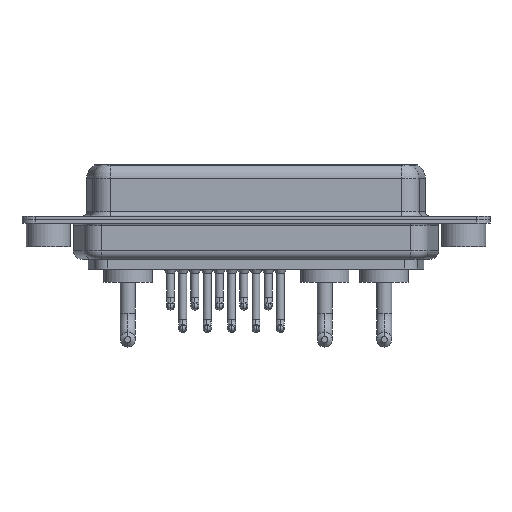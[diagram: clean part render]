
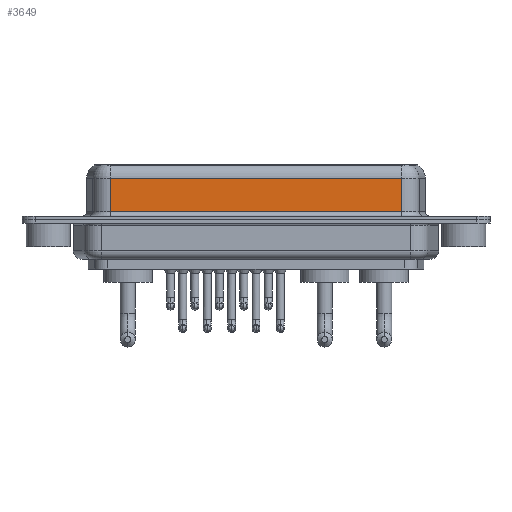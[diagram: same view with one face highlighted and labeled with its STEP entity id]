
A CAD part, front view. The second image highlights one B-rep face of the part: STEP entity #3649.
In plain terms, the highlighted planar face has unit normal (0, -1, 0).
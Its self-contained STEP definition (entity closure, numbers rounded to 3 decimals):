
#179 = LINE ( 'NONE', #17613, #16798 ) ;
#196 = VERTEX_POINT ( 'NONE', #9562 ) ;
#978 = CARTESIAN_POINT ( 'NONE',  ( 40.037, -3.95, 6.4 ) ) ;
#1635 = CARTESIAN_POINT ( 'NONE',  ( 40.037, -3.95, 4.65 ) ) ;
#2036 = ORIENTED_EDGE ( 'NONE', *, *, #8078, .T. ) ;
#2065 = ORIENTED_EDGE ( 'NONE', *, *, #15577, .F. ) ;
#2569 = CARTESIAN_POINT ( 'NONE',  ( 40.037, -3.95, 0.9 ) ) ;
#3183 = VECTOR ( 'NONE', #7528, 1000. ) ;
#3245 = EDGE_CURVE ( 'NONE', #16945, #6229, #15937, .T. ) ;
#3649 = ADVANCED_FACE ( 'NONE', ( #14176 ), #4058, .F. ) ;
#3755 = EDGE_CURVE ( 'NONE', #196, #16945, #179, .T. ) ;
#4058 = PLANE ( 'NONE',  #8174 ) ;
#5156 = ORIENTED_EDGE ( 'NONE', *, *, #3245, .T. ) ;
#5702 = VECTOR ( 'NONE', #10229, 1000. ) ;
#6049 = CARTESIAN_POINT ( 'NONE',  ( 7.013, -3.95, 0.9 ) ) ;
#6229 = VERTEX_POINT ( 'NONE', #11661 ) ;
#7528 = DIRECTION ( 'NONE',  ( -1., 0., 0. ) ) ;
#7836 = EDGE_LOOP ( 'NONE', ( #2065, #2036, #14920, #5156 ) ) ;
#8078 = EDGE_CURVE ( 'NONE', #16025, #196, #14815, .T. ) ;
#8093 = VECTOR ( 'NONE', #15496, 1000. ) ;
#8173 = CARTESIAN_POINT ( 'NONE',  ( 40.037, -3.95, 6.4 ) ) ;
#8174 = AXIS2_PLACEMENT_3D ( 'NONE', #978, #17239, #17705 ) ;
#8360 = LINE ( 'NONE', #8173, #8093 ) ;
#9494 = CARTESIAN_POINT ( 'NONE',  ( 40.037, -3.95, 4.65 ) ) ;
#9562 = CARTESIAN_POINT ( 'NONE',  ( 7.013, -3.95, 4.65 ) ) ;
#10229 = DIRECTION ( 'NONE',  ( 1., 0., 0. ) ) ;
#11661 = CARTESIAN_POINT ( 'NONE',  ( 40.037, -3.95, 0.9 ) ) ;
#14176 = FACE_OUTER_BOUND ( 'NONE', #7836, .T. ) ;
#14815 = LINE ( 'NONE', #1635, #3183 ) ;
#14920 = ORIENTED_EDGE ( 'NONE', *, *, #3755, .T. ) ;
#15496 = DIRECTION ( 'NONE',  ( 0., 0., -1. ) ) ;
#15577 = EDGE_CURVE ( 'NONE', #16025, #6229, #8360, .T. ) ;
#15937 = LINE ( 'NONE', #2569, #5702 ) ;
#16025 = VERTEX_POINT ( 'NONE', #9494 ) ;
#16798 = VECTOR ( 'NONE', #17429, 1000. ) ;
#16945 = VERTEX_POINT ( 'NONE', #6049 ) ;
#17239 = DIRECTION ( 'NONE',  ( 0., 1., 0. ) ) ;
#17429 = DIRECTION ( 'NONE',  ( 0., 0., -1. ) ) ;
#17613 = CARTESIAN_POINT ( 'NONE',  ( 7.013, -3.95, 6.4 ) ) ;
#17705 = DIRECTION ( 'NONE',  ( 0., 0., 1. ) ) ;
